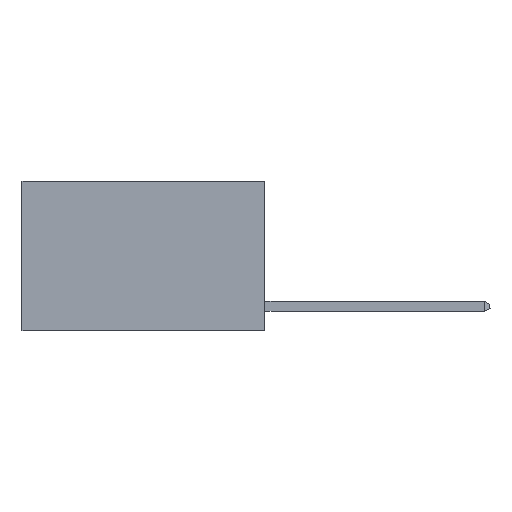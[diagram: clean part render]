
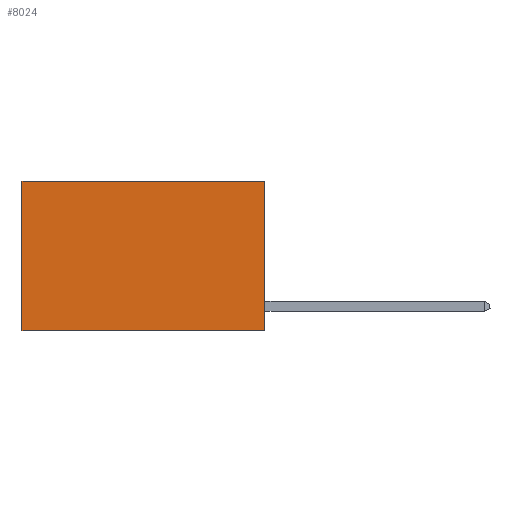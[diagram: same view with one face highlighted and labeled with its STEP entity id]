
A CAD part, left-side view. The second image highlights one B-rep face of the part: STEP entity #8024.
In plain terms, the highlighted planar face has unit normal (-1, 0, 0).
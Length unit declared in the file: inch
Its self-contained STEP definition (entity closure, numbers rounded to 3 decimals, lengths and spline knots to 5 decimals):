
#618 = ORIENTED_EDGE ( 'NONE', *, *, #14233, .T. ) ;
#708 = LINE ( 'NONE', #10995, #7205 ) ;
#755 = VECTOR ( 'NONE', #10579, 39.37008 ) ;
#1446 = DIRECTION ( 'NONE',  ( 0., 1., 0. ) ) ;
#2063 = EDGE_CURVE ( 'NONE', #11126, #16618, #7266, .T. ) ;
#2319 = CARTESIAN_POINT ( 'NONE',  ( 0.2625, 0., 0. ) ) ;
#2597 = CARTESIAN_POINT ( 'NONE',  ( 0.2625, 0., 0. ) ) ;
#2895 = VERTEX_POINT ( 'NONE', #5514 ) ;
#2919 = DIRECTION ( 'NONE',  ( 0., 0., -1. ) ) ;
#4431 = LINE ( 'NONE', #5157, #755 ) ;
#4648 = PLANE ( 'NONE',  #11957 ) ;
#5079 = ORIENTED_EDGE ( 'NONE', *, *, #2063, .F. ) ;
#5157 = CARTESIAN_POINT ( 'NONE',  ( 0.2625, 0., -0.37 ) ) ;
#5356 = LINE ( 'NONE', #9124, #15008 ) ;
#5514 = CARTESIAN_POINT ( 'NONE',  ( 0.2625, 0.6, -0.37 ) ) ;
#5851 = VERTEX_POINT ( 'NONE', #7490 ) ;
#5995 = DIRECTION ( 'NONE',  ( 0., 0., -1. ) ) ;
#6615 = ORIENTED_EDGE ( 'NONE', *, *, #9402, .F. ) ;
#7205 = VECTOR ( 'NONE', #1446, 39.37008 ) ;
#7266 = LINE ( 'NONE', #2319, #17025 ) ;
#7373 = CARTESIAN_POINT ( 'NONE',  ( 0.2625, 0., 0. ) ) ;
#7490 = CARTESIAN_POINT ( 'NONE',  ( 0.2625, 0.6, 0. ) ) ;
#8024 = ADVANCED_FACE ( 'NONE', ( #13405 ), #4648, .F. ) ;
#9124 = CARTESIAN_POINT ( 'NONE',  ( 0.2625, 0.6, 0. ) ) ;
#9402 = EDGE_CURVE ( 'NONE', #16618, #2895, #4431, .T. ) ;
#9687 = EDGE_LOOP ( 'NONE', ( #618, #6615, #5079, #11736 ) ) ;
#10551 = EDGE_CURVE ( 'NONE', #11126, #5851, #708, .T. ) ;
#10579 = DIRECTION ( 'NONE',  ( 0., 1., 0. ) ) ;
#10995 = CARTESIAN_POINT ( 'NONE',  ( 0.2625, 0., 0. ) ) ;
#11126 = VERTEX_POINT ( 'NONE', #2597 ) ;
#11736 = ORIENTED_EDGE ( 'NONE', *, *, #10551, .T. ) ;
#11957 = AXIS2_PLACEMENT_3D ( 'NONE', #7373, #13889, #5995 ) ;
#13405 = FACE_OUTER_BOUND ( 'NONE', #9687, .T. ) ;
#13889 = DIRECTION ( 'NONE',  ( 1., 0., 0. ) ) ;
#14233 = EDGE_CURVE ( 'NONE', #5851, #2895, #5356, .T. ) ;
#15008 = VECTOR ( 'NONE', #16667, 39.37008 ) ;
#16002 = CARTESIAN_POINT ( 'NONE',  ( 0.2625, 0., -0.37 ) ) ;
#16618 = VERTEX_POINT ( 'NONE', #16002 ) ;
#16667 = DIRECTION ( 'NONE',  ( 0., 0., -1. ) ) ;
#17025 = VECTOR ( 'NONE', #2919, 39.37008 ) ;
